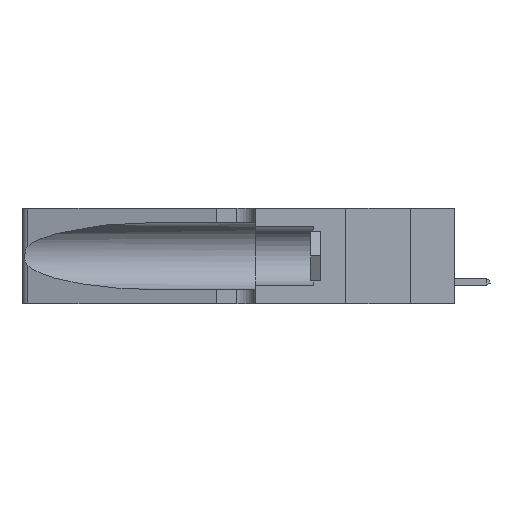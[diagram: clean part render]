
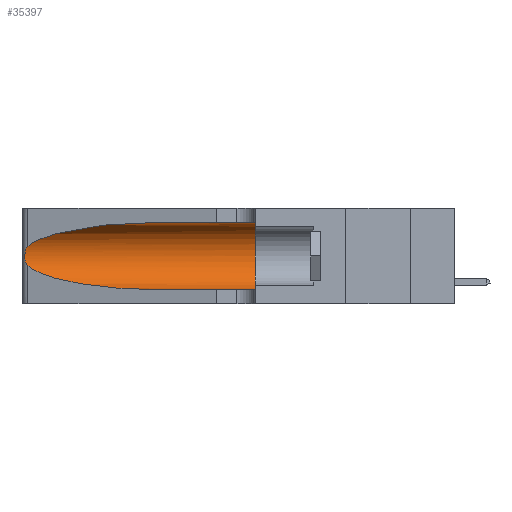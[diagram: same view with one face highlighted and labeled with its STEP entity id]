
A CAD part, left-side view. The second image highlights one B-rep face of the part: STEP entity #35397.
In plain terms, the highlighted cylindrical face has radius 3.308 mm (diameter 6.617 mm), a partial arc.
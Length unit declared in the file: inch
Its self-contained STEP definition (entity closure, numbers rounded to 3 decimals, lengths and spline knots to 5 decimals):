
#62 = ORIENTED_EDGE ( 'NONE', *, *, #32235, .F. ) ;
#102 = VERTEX_POINT ( 'NONE', #3277 ) ;
#1391 = CARTESIAN_POINT ( 'NONE',  ( 0.18966, 0.96281, 0.31525 ) ) ;
#1609 = EDGE_CURVE ( 'NONE', #102, #23229, #16116, .T. ) ;
#2913 = ORIENTED_EDGE ( 'NONE', *, *, #19209, .T. ) ;
#3064 = CARTESIAN_POINT ( 'NONE',  ( 0.25487, 1.22718, 0.14631 ) ) ;
#3277 = CARTESIAN_POINT ( 'NONE',  ( 0.1305, 0.72297, 0.31525 ) ) ;
#3317 = CARTESIAN_POINT ( 'NONE',  ( 0.18966, 0.96281, 0.05475 ) ) ;
#4040 = CARTESIAN_POINT ( 'NONE',  ( 0.25487, 1.22718, 0.22369 ) ) ;
#4053 = ORIENTED_EDGE ( 'NONE', *, *, #23725, .T. ) ;
#4185 = CARTESIAN_POINT ( 'NONE',  ( 0.25487, 1.22718, 0.22369 ) ) ;
#4715 = VERTEX_POINT ( 'NONE', #20066 ) ;
#5336 = CARTESIAN_POINT ( 'NONE',  ( 0.26075, 1.23896, 0.19203 ) ) ;
#6542 = LINE ( 'NONE', #17781, #28393 ) ;
#6904 = AXIS2_PLACEMENT_3D ( 'NONE', #27697, #13294, #7618 ) ;
#7618 = DIRECTION ( 'NONE',  ( 0., 0., 1. ) ) ;
#10986 = CARTESIAN_POINT ( 'NONE',  ( 0.26018, 1.23835, 0.19895 ) ) ;
#11230 = CARTESIAN_POINT ( 'NONE',  ( 0.25854, 1.2359, 0.20912 ) ) ;
#12872 = AXIS2_PLACEMENT_3D ( 'NONE', #30736, #27943, #24782 ) ;
#13294 = DIRECTION ( 'NONE',  ( 0., 1., 0. ) ) ;
#13800 = CARTESIAN_POINT ( 'NONE',  ( 0.25787, 1.23484, 0.2124 ) ) ;
#14030 = CARTESIAN_POINT ( 'NONE',  ( 0.25487, 1.22718, 0.14631 ) ) ;
#14163 = CARTESIAN_POINT ( 'NONE',  ( 0.26075, 1.23896, 0.178 ) ) ;
#16116 = LINE ( 'NONE', #36673, #22053 ) ;
#16212 = B_SPLINE_CURVE_WITH_KNOTS ( 'NONE', 3,
 ( #21887, #22013, #24922, #13800, #11230, #10986, #5336, #14163, #22635, #34440, #25296, #19944, #37117, #14030 ),
 .UNSPECIFIED., .F., .F.,
 ( 4, 2, 2, 2, 2, 2, 4 ),
 ( 0., 0.00027, 0.00053, 0.00107, 0.0016, 0.00187, 0.00214 ),
 .UNSPECIFIED. ) ;
#16220 = ORIENTED_EDGE ( 'NONE', *, *, #23877, .T. ) ;
#17718 = CARTESIAN_POINT ( 'NONE',  ( 0.1305, 0.35, 0.31525 ) ) ;
#17781 = CARTESIAN_POINT ( 'NONE',  ( 0.1305, 1.61858, 0.05475 ) ) ;
#18121 = VERTEX_POINT ( 'NONE', #4185 ) ;
#18481 = CARTESIAN_POINT ( 'NONE',  ( 0.1305, 0.72297, 0.31525 ) ) ;
#19088 = EDGE_LOOP ( 'NONE', ( #20414, #16220, #2913, #4053, #62, #21826 ) ) ;
#19209 = EDGE_CURVE ( 'NONE', #26791, #4715, #20590, .T. ) ;
#19944 = CARTESIAN_POINT ( 'NONE',  ( 0.25639, 1.23186, 0.15144 ) ) ;
#20066 = CARTESIAN_POINT ( 'NONE',  ( 0.1305, 0.72297, 0.05475 ) ) ;
#20414 = ORIENTED_EDGE ( 'NONE', *, *, #34339, .T. ) ;
#20509 = CARTESIAN_POINT ( 'NONE',  ( 0.1305, 0.35, 0.05475 ) ) ;
#20590 =( BOUNDED_CURVE ( )  B_SPLINE_CURVE ( 3, ( #3064, #20666, #3317, #29693 ),
 .UNSPECIFIED., .F., .T. ) 
 B_SPLINE_CURVE_WITH_KNOTS ( ( 4, 4 ),
 ( 3.44316, 4.71239 ),
 .UNSPECIFIED. ) 
 CURVE ( )  GEOMETRIC_REPRESENTATION_ITEM ( )  RATIONAL_B_SPLINE_CURVE ( ( 1., 0.87, 0.87, 1. ) ) 
 REPRESENTATION_ITEM ( '' )  );
#20666 = CARTESIAN_POINT ( 'NONE',  ( 0.2373, 1.15595, 0.08982 ) ) ;
#21146 = FACE_OUTER_BOUND ( 'NONE', #19088, .T. ) ;
#21826 = ORIENTED_EDGE ( 'NONE', *, *, #1609, .F. ) ;
#21887 = CARTESIAN_POINT ( 'NONE',  ( 0.25487, 1.22718, 0.22369 ) ) ;
#22013 = CARTESIAN_POINT ( 'NONE',  ( 0.25555, 1.22994, 0.2215 ) ) ;
#22053 = VECTOR ( 'NONE', #28146, 39.37008 ) ;
#22635 = CARTESIAN_POINT ( 'NONE',  ( 0.26017, 1.23833, 0.17102 ) ) ;
#22847 = CIRCLE ( 'NONE', #6904, 0.13025 ) ;
#23229 = VERTEX_POINT ( 'NONE', #17718 ) ;
#23725 = EDGE_CURVE ( 'NONE', #4715, #29672, #6542, .T. ) ;
#23877 = EDGE_CURVE ( 'NONE', #18121, #26791, #16212, .T. ) ;
#24223 = CARTESIAN_POINT ( 'NONE',  ( 0.2373, 1.15595, 0.28018 ) ) ;
#24782 = DIRECTION ( 'NONE',  ( 0., 0., -1. ) ) ;
#24922 = CARTESIAN_POINT ( 'NONE',  ( 0.25639, 1.23184, 0.21858 ) ) ;
#25296 = CARTESIAN_POINT ( 'NONE',  ( 0.25789, 1.23486, 0.15765 ) ) ;
#26791 = VERTEX_POINT ( 'NONE', #29046 ) ;
#27697 = CARTESIAN_POINT ( 'NONE',  ( 0.1305, 0.35, 0.185 ) ) ;
#27943 = DIRECTION ( 'NONE',  ( 0., -1., 0. ) ) ;
#28146 = DIRECTION ( 'NONE',  ( 0., -1., 0. ) ) ;
#28393 = VECTOR ( 'NONE', #29463, 39.37008 ) ;
#29046 = CARTESIAN_POINT ( 'NONE',  ( 0.25487, 1.22718, 0.14631 ) ) ;
#29463 = DIRECTION ( 'NONE',  ( 0., -1., 0. ) ) ;
#29672 = VERTEX_POINT ( 'NONE', #20509 ) ;
#29693 = CARTESIAN_POINT ( 'NONE',  ( 0.1305, 0.72297, 0.05475 ) ) ;
#29787 = CYLINDRICAL_SURFACE ( 'NONE', #12872, 0.13025 ) ;
#30736 = CARTESIAN_POINT ( 'NONE',  ( 0.1305, 1.61858, 0.185 ) ) ;
#32235 = EDGE_CURVE ( 'NONE', #23229, #29672, #22847, .T. ) ;
#32484 =( BOUNDED_CURVE ( )  B_SPLINE_CURVE ( 3, ( #18481, #1391, #24223, #4040 ),
 .UNSPECIFIED., .F., .F. ) 
 B_SPLINE_CURVE_WITH_KNOTS ( ( 4, 4 ),
 ( 1.5708, 2.84003 ),
 .UNSPECIFIED. ) 
 CURVE ( )  GEOMETRIC_REPRESENTATION_ITEM ( )  RATIONAL_B_SPLINE_CURVE ( ( 1., 0.87, 0.87, 1. ) ) 
 REPRESENTATION_ITEM ( '' )  );
#34339 = EDGE_CURVE ( 'NONE', #102, #18121, #32484, .T. ) ;
#34440 = CARTESIAN_POINT ( 'NONE',  ( 0.25856, 1.23593, 0.16098 ) ) ;
#35397 = ADVANCED_FACE ( 'NONE', ( #21146 ), #29787, .F. ) ;
#36673 = CARTESIAN_POINT ( 'NONE',  ( 0.1305, 1.61858, 0.31525 ) ) ;
#37117 = CARTESIAN_POINT ( 'NONE',  ( 0.25555, 1.22993, 0.14849 ) ) ;
